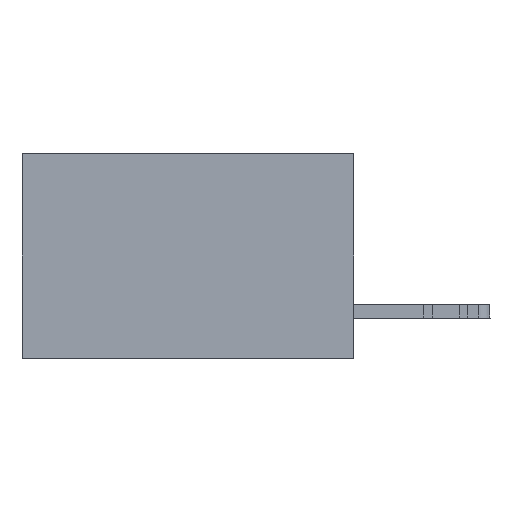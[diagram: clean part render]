
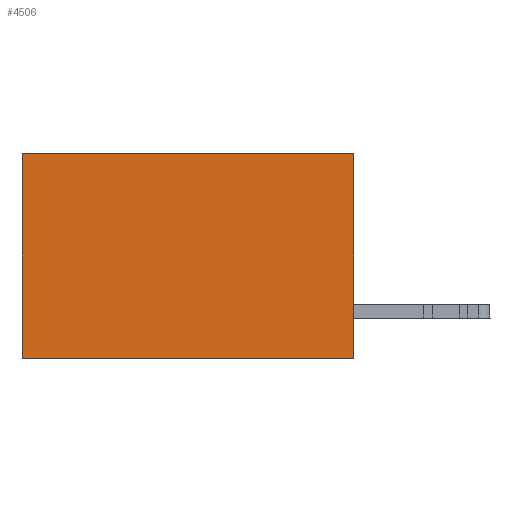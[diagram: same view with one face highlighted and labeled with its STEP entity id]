
A CAD part, left-side view. The second image highlights one B-rep face of the part: STEP entity #4506.
In plain terms, the highlighted planar face has unit normal (-1, 0, 0).
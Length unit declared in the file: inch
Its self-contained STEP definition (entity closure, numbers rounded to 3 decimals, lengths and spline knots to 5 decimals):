
#293 = VECTOR ( 'NONE', #16130, 39.37008 ) ;
#3884 = EDGE_CURVE ( 'NONE', #45730, #35892, #20099, .T. ) ;
#4506 = ADVANCED_FACE ( 'NONE', ( #5826 ), #8617, .F. ) ;
#5826 = FACE_OUTER_BOUND ( 'NONE', #9972, .T. ) ;
#6978 = CARTESIAN_POINT ( 'NONE',  ( 0.2875, 0.6, 0. ) ) ;
#8170 = DIRECTION ( 'NONE',  ( 0., 0., -1. ) ) ;
#8617 = PLANE ( 'NONE',  #31167 ) ;
#9879 = EDGE_CURVE ( 'NONE', #35892, #28763, #17738, .T. ) ;
#9972 = EDGE_LOOP ( 'NONE', ( #46548, #45834, #30218, #37999 ) ) ;
#11850 = DIRECTION ( 'NONE',  ( 1., 0., 0. ) ) ;
#12616 = DIRECTION ( 'NONE',  ( 0., 0., -1. ) ) ;
#14146 = VECTOR ( 'NONE', #21398, 39.37008 ) ;
#14544 = VERTEX_POINT ( 'NONE', #25507 ) ;
#15820 = LINE ( 'NONE', #46267, #293 ) ;
#16130 = DIRECTION ( 'NONE',  ( 0., 1., 0. ) ) ;
#16556 = LINE ( 'NONE', #6978, #29788 ) ;
#17738 = LINE ( 'NONE', #39831, #14146 ) ;
#20099 = LINE ( 'NONE', #23699, #36129 ) ;
#21398 = DIRECTION ( 'NONE',  ( 0., 1., 0. ) ) ;
#21942 = CARTESIAN_POINT ( 'NONE',  ( 0.2875, 0., 0. ) ) ;
#23699 = CARTESIAN_POINT ( 'NONE',  ( 0.2875, 0., 0. ) ) ;
#25507 = CARTESIAN_POINT ( 'NONE',  ( 0.2875, 0.6, 0. ) ) ;
#26415 = DIRECTION ( 'NONE',  ( 0., 0., -1. ) ) ;
#26685 = EDGE_CURVE ( 'NONE', #45730, #14544, #15820, .T. ) ;
#28284 = CARTESIAN_POINT ( 'NONE',  ( 0.2875, 0., -0.37 ) ) ;
#28763 = VERTEX_POINT ( 'NONE', #31129 ) ;
#29788 = VECTOR ( 'NONE', #26415, 39.37008 ) ;
#30218 = ORIENTED_EDGE ( 'NONE', *, *, #3884, .F. ) ;
#31129 = CARTESIAN_POINT ( 'NONE',  ( 0.2875, 0.6, -0.37 ) ) ;
#31167 = AXIS2_PLACEMENT_3D ( 'NONE', #46257, #11850, #8170 ) ;
#35892 = VERTEX_POINT ( 'NONE', #28284 ) ;
#36129 = VECTOR ( 'NONE', #12616, 39.37008 ) ;
#37999 = ORIENTED_EDGE ( 'NONE', *, *, #26685, .T. ) ;
#39831 = CARTESIAN_POINT ( 'NONE',  ( 0.2875, 0., -0.37 ) ) ;
#45730 = VERTEX_POINT ( 'NONE', #21942 ) ;
#45834 = ORIENTED_EDGE ( 'NONE', *, *, #9879, .F. ) ;
#46257 = CARTESIAN_POINT ( 'NONE',  ( 0.2875, 0., 0. ) ) ;
#46267 = CARTESIAN_POINT ( 'NONE',  ( 0.2875, 0., 0. ) ) ;
#46548 = ORIENTED_EDGE ( 'NONE', *, *, #47630, .T. ) ;
#47630 = EDGE_CURVE ( 'NONE', #14544, #28763, #16556, .T. ) ;
